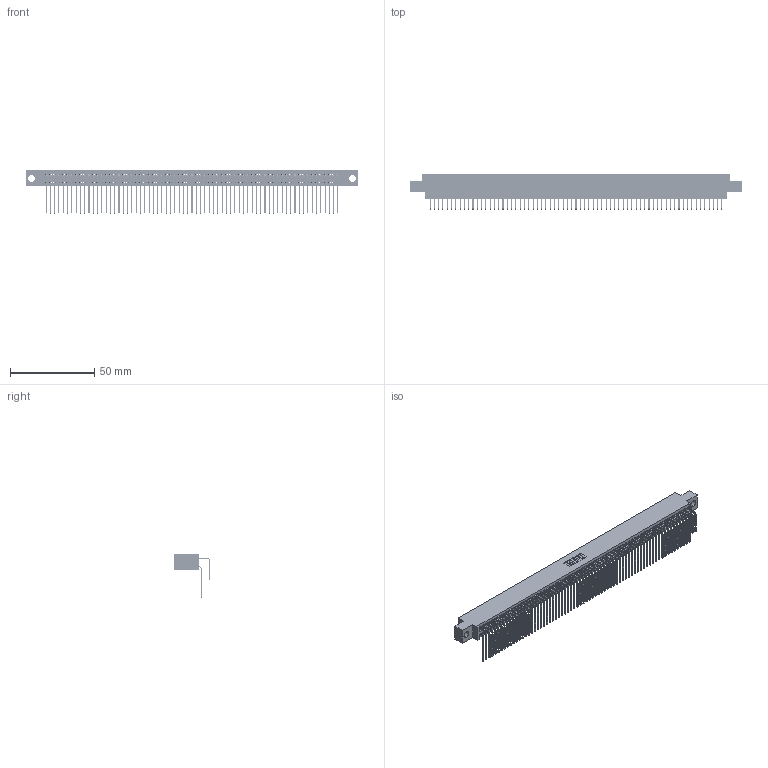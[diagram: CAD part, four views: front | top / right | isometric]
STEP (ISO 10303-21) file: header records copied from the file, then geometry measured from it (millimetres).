
FILE_DESCRIPTION (( 'STEP AP203' ), '1' );
FILE_NAME ('395-138-558-804.STEP', '2018-12-05T17:51:37', ( '' ), ( '' ), 'SwSTEP 2.0', 'SolidWorks 2016', '' );
FILE_SCHEMA (( 'CONFIG_CONTROL_DESIGN' ));
Length unit declared in the file: inch
Products named in the file (4): 345-292-001_558 Tail - 2; 395-138-558-804; 345-292-001_558 559 Tail - 1; 345 Part_0.170 Offset - 0.156 Dia-TH
Assembly tree (139 placements, depth 2):
  395-138-558-804
    345 Part_0.170 Offset - 0.156 Dia-TH
    345-292-001_558 559 Tail - 1  x69
    345-292-001_558 Tail - 2  x69
Bounding box: 196.47 x 21.83 x 25.53 mm (x, y, z)
Volume: 19930.7 mm3; surface area: 33685.9 mm2
Topology: 139 solids, 139 shells, 7306 faces, 21743 edges, 14310 vertices
Faces by surface type: plane 4914, cylinder 2392
Entity records: 52291 total; most frequent: CARTESIAN_POINT 8787, ORIENTED_EDGE 8670, DIRECTION 7687, EDGE_CURVE 4335, LINE 3887, VECTOR 3887, VERTEX_POINT 2886, AXIS2_PLACEMENT_3D 1900
